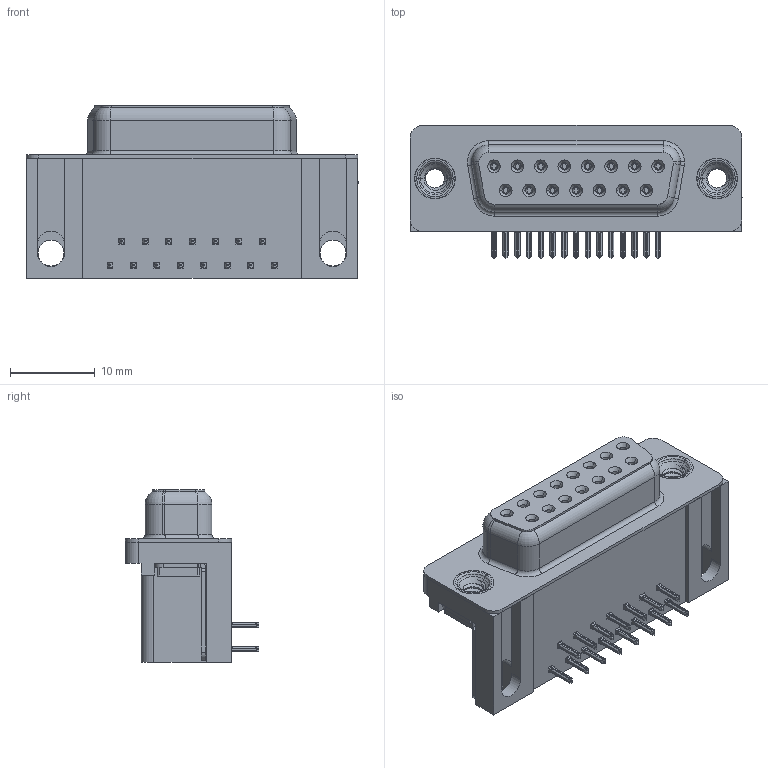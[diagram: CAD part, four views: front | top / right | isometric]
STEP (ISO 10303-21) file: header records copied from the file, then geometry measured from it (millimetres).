
FILE_DESCRIPTION (( 'STEP AP203' ), '1' );
FILE_NAME ('630-015-240-012.STEP', '2021-09-22T13:29:11', ( '' ), ( '' ), 'SwSTEP 2.0', 'SolidWorks 2020', '' );
FILE_SCHEMA (( 'CONFIG_CONTROL_DESIGN' ));
Length unit declared in the file: millimetre
Products named in the file (7): 630 Contact Bottom; 630 Contact Top; 630 Thru Hole Board Mount; 630 Housing_15 Socket; 630-015-240-012; 630 4-40 Threaded Rivet; 630 Shell_15 Socket
Assembly tree (21 placements, depth 2):
  630-015-240-012
    630 Housing_15 Socket
    630 Shell_15 Socket
    630 Contact Bottom  x7
    630 Contact Top  x8
    630 Thru Hole Board Mount  x2
    630 4-40 Threaded Rivet  x2
Bounding box: 39.22 x 15.73 x 20.4 mm (x, y, z)
Volume: 5855.8 mm3; surface area: 7167.4 mm2
Topology: 21 solids, 21 shells, 2425 faces, 6364 edges, 3996 vertices
Faces by surface type: plane 1072, cylinder 605, bspline 518, cone 192, torus 38
Entity records: 26461 total; most frequent: CARTESIAN_POINT 8983, ORIENTED_EDGE 3532, DIRECTION 3154, EDGE_CURVE 1766, VERTEX_POINT 1124, LINE 1086, VECTOR 1086, AXIS2_PLACEMENT_3D 1034
